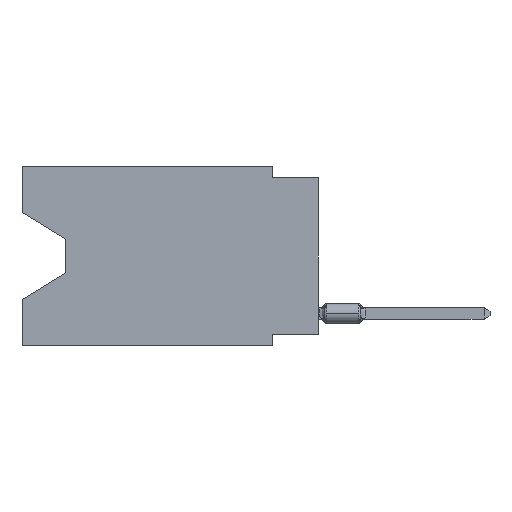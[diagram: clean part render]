
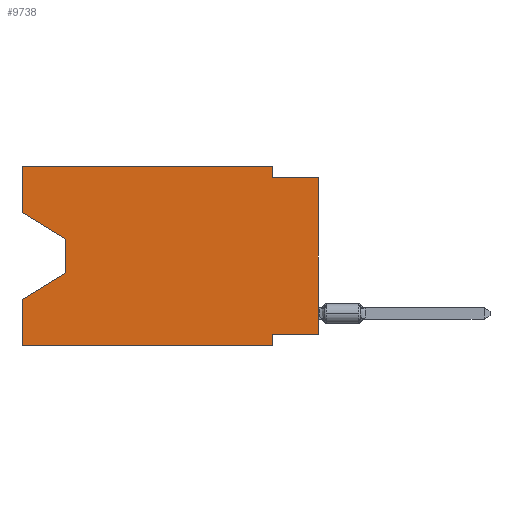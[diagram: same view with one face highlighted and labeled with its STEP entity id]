
A CAD part, left-side view. The second image highlights one B-rep face of the part: STEP entity #9738.
In plain terms, the highlighted planar face has unit normal (-1, 0, 0).
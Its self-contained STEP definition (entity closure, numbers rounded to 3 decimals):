
#186 = EDGE_CURVE ( 'NONE', #1814, #7585, #12347, .T. ) ;
#585 = VERTEX_POINT ( 'NONE', #9757 ) ;
#1259 = ORIENTED_EDGE ( 'NONE', *, *, #16188, .F. ) ;
#1344 = VECTOR ( 'NONE', #20936, 1000. ) ;
#1525 = EDGE_LOOP ( 'NONE', ( #14347, #16526, #9854, #1259, #11275, #10241, #8184, #16029, #19188, #18535, #22379, #14819 ) ) ;
#1814 = VERTEX_POINT ( 'NONE', #5694 ) ;
#1986 = VECTOR ( 'NONE', #9495, 1000. ) ;
#2950 = LINE ( 'NONE', #17956, #4001 ) ;
#3196 = DIRECTION ( 'NONE',  ( 1., 0., 0. ) ) ;
#3375 = CARTESIAN_POINT ( 'NONE',  ( 0., 16.383, 0. ) ) ;
#3597 = VECTOR ( 'NONE', #8615, 1000. ) ;
#3611 = EDGE_CURVE ( 'NONE', #17092, #10463, #9257, .T. ) ;
#3968 = CARTESIAN_POINT ( 'NONE',  ( 0., 0., -0.635 ) ) ;
#4001 = VECTOR ( 'NONE', #10280, 1000. ) ;
#4460 = LINE ( 'NONE', #16833, #1344 ) ;
#4782 = DIRECTION ( 'NONE',  ( 0., 0., 1. ) ) ;
#4844 = CARTESIAN_POINT ( 'NONE',  ( 0., 2.54, -9.906 ) ) ;
#5031 = VERTEX_POINT ( 'NONE', #3968 ) ;
#5116 = DIRECTION ( 'NONE',  ( 0., 0., -1. ) ) ;
#5417 = DIRECTION ( 'NONE',  ( 0., -1., 0. ) ) ;
#5694 = CARTESIAN_POINT ( 'NONE',  ( 0., 0., -9.271 ) ) ;
#5937 = DIRECTION ( 'NONE',  ( 0., -1., 0. ) ) ;
#6083 = CARTESIAN_POINT ( 'NONE',  ( 0., 2.54, -0.635 ) ) ;
#6163 = VECTOR ( 'NONE', #5937, 1000. ) ;
#6817 = LINE ( 'NONE', #10311, #19063 ) ;
#6984 = DIRECTION ( 'NONE',  ( 0., 0., 1. ) ) ;
#7100 = CARTESIAN_POINT ( 'NONE',  ( 0., 2.54, 0. ) ) ;
#7228 = CARTESIAN_POINT ( 'NONE',  ( 0., 16.383, 0. ) ) ;
#7289 = VERTEX_POINT ( 'NONE', #20962 ) ;
#7409 = CARTESIAN_POINT ( 'NONE',  ( 0., 16.383, -9.906 ) ) ;
#7585 = VERTEX_POINT ( 'NONE', #20327 ) ;
#8184 = ORIENTED_EDGE ( 'NONE', *, *, #186, .F. ) ;
#8615 = DIRECTION ( 'NONE',  ( 0., 1., 0. ) ) ;
#8714 = VERTEX_POINT ( 'NONE', #6083 ) ;
#8823 = VECTOR ( 'NONE', #20387, 1000. ) ;
#9257 = LINE ( 'NONE', #16585, #11996 ) ;
#9495 = DIRECTION ( 'NONE',  ( 0., 0., 1. ) ) ;
#9566 = CARTESIAN_POINT ( 'NONE',  ( 0., 2.54, 0. ) ) ;
#9615 = CARTESIAN_POINT ( 'NONE',  ( 0., 16.383, 0. ) ) ;
#9738 = ADVANCED_FACE ( 'NONE', ( #16280 ), #19649, .F. ) ;
#9757 = CARTESIAN_POINT ( 'NONE',  ( 0., 13.97, -4.013 ) ) ;
#9854 = ORIENTED_EDGE ( 'NONE', *, *, #20634, .T. ) ;
#10241 = ORIENTED_EDGE ( 'NONE', *, *, #21421, .F. ) ;
#10280 = DIRECTION ( 'NONE',  ( 0., -1., 0. ) ) ;
#10311 = CARTESIAN_POINT ( 'NONE',  ( 0., 0., 0. ) ) ;
#10359 = VERTEX_POINT ( 'NONE', #7228 ) ;
#10463 = VERTEX_POINT ( 'NONE', #10496 ) ;
#10483 = LINE ( 'NONE', #7100, #19182 ) ;
#10496 = CARTESIAN_POINT ( 'NONE',  ( 0., 2.54, -9.906 ) ) ;
#10593 = LINE ( 'NONE', #3375, #23470 ) ;
#10697 = LINE ( 'NONE', #16100, #13864 ) ;
#10764 = EDGE_CURVE ( 'NONE', #585, #12741, #10697, .T. ) ;
#10832 = DIRECTION ( 'NONE',  ( 0., 0., -1. ) ) ;
#11275 = ORIENTED_EDGE ( 'NONE', *, *, #3611, .T. ) ;
#11278 = CARTESIAN_POINT ( 'NONE',  ( 0., 16.383, -2.546 ) ) ;
#11996 = VECTOR ( 'NONE', #5417, 1000. ) ;
#12347 = LINE ( 'NONE', #16055, #3597 ) ;
#12519 = DIRECTION ( 'NONE',  ( 0., 0., -1. ) ) ;
#12741 = VERTEX_POINT ( 'NONE', #19411 ) ;
#13238 = EDGE_CURVE ( 'NONE', #7289, #585, #22326, .T. ) ;
#13864 = VECTOR ( 'NONE', #10832, 1000. ) ;
#13885 = VERTEX_POINT ( 'NONE', #16339 ) ;
#14186 = AXIS2_PLACEMENT_3D ( 'NONE', #14375, #3196, #5116 ) ;
#14333 = EDGE_CURVE ( 'NONE', #8714, #5031, #15088, .T. ) ;
#14347 = ORIENTED_EDGE ( 'NONE', *, *, #13238, .T. ) ;
#14375 = CARTESIAN_POINT ( 'NONE',  ( 0., 16.383, 0. ) ) ;
#14819 = ORIENTED_EDGE ( 'NONE', *, *, #16327, .F. ) ;
#15088 = LINE ( 'NONE', #22421, #6163 ) ;
#16029 = ORIENTED_EDGE ( 'NONE', *, *, #18473, .T. ) ;
#16055 = CARTESIAN_POINT ( 'NONE',  ( 0., 0., -9.271 ) ) ;
#16100 = CARTESIAN_POINT ( 'NONE',  ( 0., 13.97, -4.013 ) ) ;
#16188 = EDGE_CURVE ( 'NONE', #17092, #13885, #10593, .T. ) ;
#16280 = FACE_OUTER_BOUND ( 'NONE', #1525, .T. ) ;
#16327 = EDGE_CURVE ( 'NONE', #7289, #10359, #22482, .T. ) ;
#16339 = CARTESIAN_POINT ( 'NONE',  ( 0., 16.383, -7.36 ) ) ;
#16526 = ORIENTED_EDGE ( 'NONE', *, *, #10764, .T. ) ;
#16585 = CARTESIAN_POINT ( 'NONE',  ( 0., 16.383, -9.906 ) ) ;
#16833 = CARTESIAN_POINT ( 'NONE',  ( 0., 13.97, -5.893 ) ) ;
#17092 = VERTEX_POINT ( 'NONE', #7409 ) ;
#17479 = VERTEX_POINT ( 'NONE', #9566 ) ;
#17956 = CARTESIAN_POINT ( 'NONE',  ( 0., 16.383, 0. ) ) ;
#18473 = EDGE_CURVE ( 'NONE', #1814, #5031, #6817, .T. ) ;
#18535 = ORIENTED_EDGE ( 'NONE', *, *, #21890, .F. ) ;
#19063 = VECTOR ( 'NONE', #4782, 1000. ) ;
#19142 = DIRECTION ( 'NONE',  ( 0., 0., -1. ) ) ;
#19182 = VECTOR ( 'NONE', #12519, 1000. ) ;
#19188 = ORIENTED_EDGE ( 'NONE', *, *, #14333, .F. ) ;
#19411 = CARTESIAN_POINT ( 'NONE',  ( 0., 13.97, -5.893 ) ) ;
#19649 = PLANE ( 'NONE',  #14186 ) ;
#20110 = EDGE_CURVE ( 'NONE', #10359, #17479, #2950, .T. ) ;
#20327 = CARTESIAN_POINT ( 'NONE',  ( 0., 2.54, -9.271 ) ) ;
#20387 = DIRECTION ( 'NONE',  ( 0., -0.855, -0.519 ) ) ;
#20634 = EDGE_CURVE ( 'NONE', #12741, #13885, #4460, .T. ) ;
#20936 = DIRECTION ( 'NONE',  ( 0., 0.855, -0.519 ) ) ;
#20951 = VECTOR ( 'NONE', #19142, 1000. ) ;
#20962 = CARTESIAN_POINT ( 'NONE',  ( 0., 16.383, -2.546 ) ) ;
#21084 = LINE ( 'NONE', #4844, #20951 ) ;
#21421 = EDGE_CURVE ( 'NONE', #7585, #10463, #21084, .T. ) ;
#21890 = EDGE_CURVE ( 'NONE', #17479, #8714, #10483, .T. ) ;
#22326 = LINE ( 'NONE', #11278, #8823 ) ;
#22379 = ORIENTED_EDGE ( 'NONE', *, *, #20110, .F. ) ;
#22421 = CARTESIAN_POINT ( 'NONE',  ( 0., 0., -0.635 ) ) ;
#22482 = LINE ( 'NONE', #9615, #1986 ) ;
#23470 = VECTOR ( 'NONE', #6984, 1000. ) ;
